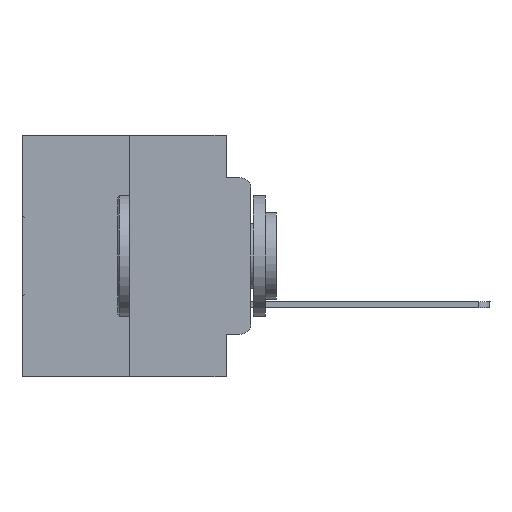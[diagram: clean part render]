
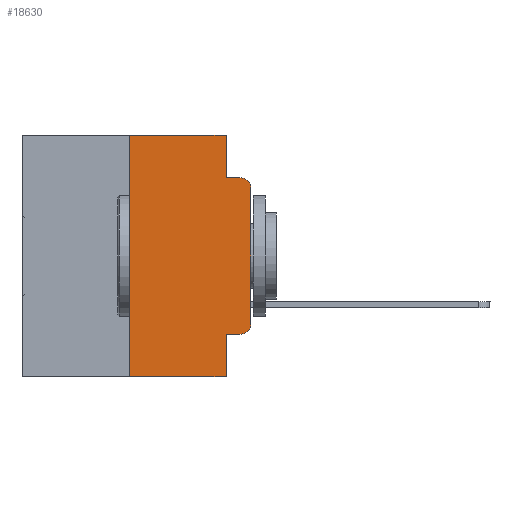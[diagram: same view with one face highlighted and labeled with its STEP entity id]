
A CAD part, left-side view. The second image highlights one B-rep face of the part: STEP entity #18630.
In plain terms, the highlighted planar face has unit normal (-1, 0, 0).
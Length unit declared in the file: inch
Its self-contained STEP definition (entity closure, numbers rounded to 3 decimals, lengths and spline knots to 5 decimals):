
#137 = ORIENTED_EDGE ( 'NONE', *, *, #13173, .T. ) ;
#215 = DIRECTION ( 'NONE',  ( 0., -1., 0. ) ) ;
#628 = CARTESIAN_POINT ( 'NONE',  ( 0., 0.473, 0. ) ) ;
#1385 = CARTESIAN_POINT ( 'NONE',  ( 0., 0.051, -0.5 ) ) ;
#1727 = DIRECTION ( 'NONE',  ( 0., 0., -1. ) ) ;
#1765 = VERTEX_POINT ( 'NONE', #5871 ) ;
#1875 = ORIENTED_EDGE ( 'NONE', *, *, #22931, .T. ) ;
#2075 = DIRECTION ( 'NONE',  ( 0., -1., 0. ) ) ;
#2488 = CIRCLE ( 'NONE', #17730, 0.02 ) ;
#2904 = ORIENTED_EDGE ( 'NONE', *, *, #15929, .T. ) ;
#3094 = VERTEX_POINT ( 'NONE', #1385 ) ;
#3438 = DIRECTION ( 'NONE',  ( 0., 0., -1. ) ) ;
#3493 = EDGE_CURVE ( 'NONE', #18916, #31352, #30098, .T. ) ;
#3631 = CARTESIAN_POINT ( 'NONE',  ( 0., 0.02, -0.0885 ) ) ;
#3774 = CARTESIAN_POINT ( 'NONE',  ( 0., 0.473, 0. ) ) ;
#3817 = AXIS2_PLACEMENT_3D ( 'NONE', #20651, #12369, #5551 ) ;
#4093 = DIRECTION ( 'NONE',  ( 0., -1., 0. ) ) ;
#4177 = VERTEX_POINT ( 'NONE', #7829 ) ;
#4450 = ORIENTED_EDGE ( 'NONE', *, *, #20549, .F. ) ;
#4671 = FACE_OUTER_BOUND ( 'NONE', #26124, .T. ) ;
#5082 = ORIENTED_EDGE ( 'NONE', *, *, #10901, .F. ) ;
#5551 = DIRECTION ( 'NONE',  ( 0., 0., -1. ) ) ;
#5871 = CARTESIAN_POINT ( 'NONE',  ( 0., 0.25, -0.5 ) ) ;
#6349 = LINE ( 'NONE', #12532, #20952 ) ;
#6820 = ORIENTED_EDGE ( 'NONE', *, *, #23453, .T. ) ;
#7582 = DIRECTION ( 'NONE',  ( 0., 0., -1. ) ) ;
#7829 = CARTESIAN_POINT ( 'NONE',  ( 0., 0.051, -0.4115 ) ) ;
#8236 = DIRECTION ( 'NONE',  ( 0., 0., 1. ) ) ;
#9020 = VECTOR ( 'NONE', #8236, 39.37008 ) ;
#9722 = CARTESIAN_POINT ( 'NONE',  ( 0., 0.02, -0.4115 ) ) ;
#10006 = CARTESIAN_POINT ( 'NONE',  ( 0., 0.051, -0.0885 ) ) ;
#10252 = VECTOR ( 'NONE', #215, 39.37008 ) ;
#10740 = DIRECTION ( 'NONE',  ( 1., 0., 0. ) ) ;
#10901 = EDGE_CURVE ( 'NONE', #1765, #21130, #17203, .T. ) ;
#11053 = LINE ( 'NONE', #10006, #10252 ) ;
#11589 = CARTESIAN_POINT ( 'NONE',  ( 0., 0.051, -0.0885 ) ) ;
#12369 = DIRECTION ( 'NONE',  ( -1., 0., 0. ) ) ;
#12532 = CARTESIAN_POINT ( 'NONE',  ( 0., 0.051, 0. ) ) ;
#12834 = PLANE ( 'NONE',  #16005 ) ;
#13173 = EDGE_CURVE ( 'NONE', #1765, #3094, #20595, .T. ) ;
#13355 = VERTEX_POINT ( 'NONE', #11589 ) ;
#14325 = EDGE_CURVE ( 'NONE', #4177, #3094, #6349, .T. ) ;
#14446 = VECTOR ( 'NONE', #25226, 39.37008 ) ;
#15929 = EDGE_CURVE ( 'NONE', #31736, #18916, #29524, .T. ) ;
#16005 = AXIS2_PLACEMENT_3D ( 'NONE', #628, #10740, #16034 ) ;
#16034 = DIRECTION ( 'NONE',  ( 0., 0., -1. ) ) ;
#16118 = CARTESIAN_POINT ( 'NONE',  ( 0., 0.051, 0. ) ) ;
#16417 = CARTESIAN_POINT ( 'NONE',  ( 0., 0.25, 0. ) ) ;
#16549 = EDGE_CURVE ( 'NONE', #21863, #13355, #27455, .T. ) ;
#17014 = ORIENTED_EDGE ( 'NONE', *, *, #3493, .T. ) ;
#17203 = LINE ( 'NONE', #28298, #14446 ) ;
#17730 = AXIS2_PLACEMENT_3D ( 'NONE', #22307, #24649, #1727 ) ;
#17834 = EDGE_CURVE ( 'NONE', #13355, #31352, #11053, .T. ) ;
#18282 = DIRECTION ( 'NONE',  ( 0., -1., 0. ) ) ;
#18630 = ADVANCED_FACE ( 'NONE', ( #4671 ), #12834, .F. ) ;
#18916 = VERTEX_POINT ( 'NONE', #19635 ) ;
#19635 = CARTESIAN_POINT ( 'NONE',  ( 0., 0., -0.1085 ) ) ;
#19806 = ORIENTED_EDGE ( 'NONE', *, *, #14325, .F. ) ;
#20157 = CARTESIAN_POINT ( 'NONE',  ( 0., 0.051, -0.4115 ) ) ;
#20549 = EDGE_CURVE ( 'NONE', #21130, #21863, #31473, .T. ) ;
#20595 = LINE ( 'NONE', #23631, #31635 ) ;
#20651 = CARTESIAN_POINT ( 'NONE',  ( 0., 0.02, -0.1085 ) ) ;
#20952 = VECTOR ( 'NONE', #7582, 39.37008 ) ;
#21130 = VERTEX_POINT ( 'NONE', #16417 ) ;
#21863 = VERTEX_POINT ( 'NONE', #26629 ) ;
#21991 = ORIENTED_EDGE ( 'NONE', *, *, #17834, .F. ) ;
#22307 = CARTESIAN_POINT ( 'NONE',  ( 0., 0.02, -0.3915 ) ) ;
#22931 = EDGE_CURVE ( 'NONE', #4177, #25404, #24417, .T. ) ;
#23453 = EDGE_CURVE ( 'NONE', #25404, #31736, #2488, .T. ) ;
#23631 = CARTESIAN_POINT ( 'NONE',  ( 0., 0.473, -0.5 ) ) ;
#24417 = LINE ( 'NONE', #20157, #31502 ) ;
#24649 = DIRECTION ( 'NONE',  ( -1., 0., 0. ) ) ;
#24730 = ORIENTED_EDGE ( 'NONE', *, *, #16549, .F. ) ;
#25226 = DIRECTION ( 'NONE',  ( 0., 0., 1. ) ) ;
#25404 = VERTEX_POINT ( 'NONE', #9722 ) ;
#26124 = EDGE_LOOP ( 'NONE', ( #2904, #17014, #21991, #24730, #4450, #5082, #137, #19806, #1875, #6820 ) ) ;
#26195 = CARTESIAN_POINT ( 'NONE',  ( 0., 0., 0. ) ) ;
#26629 = CARTESIAN_POINT ( 'NONE',  ( 0., 0.051, 0. ) ) ;
#27455 = LINE ( 'NONE', #16118, #28651 ) ;
#28298 = CARTESIAN_POINT ( 'NONE',  ( 0., 0.25, 0. ) ) ;
#28651 = VECTOR ( 'NONE', #3438, 39.37008 ) ;
#29524 = LINE ( 'NONE', #26195, #9020 ) ;
#30098 = CIRCLE ( 'NONE', #3817, 0.02 ) ;
#30280 = VECTOR ( 'NONE', #4093, 39.37008 ) ;
#30524 = CARTESIAN_POINT ( 'NONE',  ( 0., 0., -0.3915 ) ) ;
#31352 = VERTEX_POINT ( 'NONE', #3631 ) ;
#31473 = LINE ( 'NONE', #3774, #30280 ) ;
#31502 = VECTOR ( 'NONE', #2075, 39.37008 ) ;
#31635 = VECTOR ( 'NONE', #18282, 39.37008 ) ;
#31736 = VERTEX_POINT ( 'NONE', #30524 ) ;
